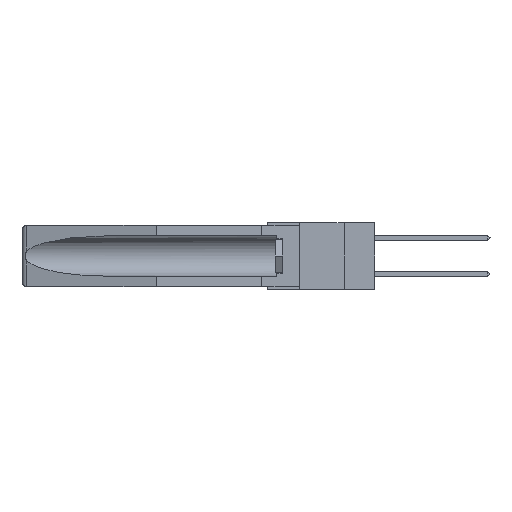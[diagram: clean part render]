
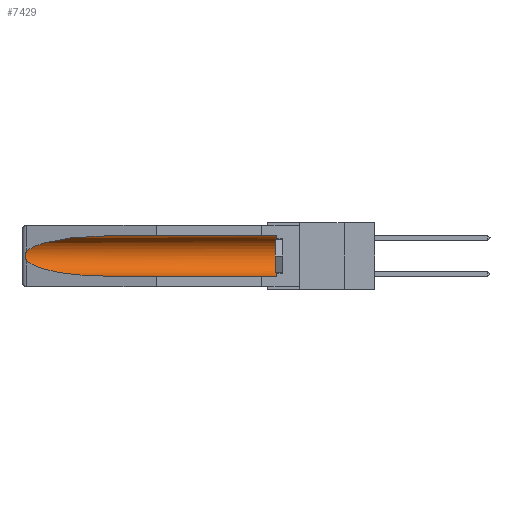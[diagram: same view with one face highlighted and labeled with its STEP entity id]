
A CAD part, left-side view. The second image highlights one B-rep face of the part: STEP entity #7429.
In plain terms, the highlighted cylindrical face has radius 2.857 mm (diameter 5.715 mm), a partial arc.
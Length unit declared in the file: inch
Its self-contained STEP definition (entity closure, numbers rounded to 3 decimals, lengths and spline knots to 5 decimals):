
#941 = DIRECTION ( 'NONE',  ( 0., 0., 1. ) ) ;
#954 = B_SPLINE_CURVE_WITH_KNOTS ( 'NONE', 3,
 ( #19045, #12262, #14741, #13070, #11184, #18297, #9565, #6142, #7768, #18066 ),
 .UNSPECIFIED., .F., .F.,
 ( 4, 2, 2, 2, 4 ),
 ( 0., 0.00029, 0.00058, 0.00087, 0.00117 ),
 .UNSPECIFIED. ) ;
#1592 = FACE_OUTER_BOUND ( 'NONE', #9227, .T. ) ;
#1776 = VECTOR ( 'NONE', #9390, 39.37008 ) ;
#2750 = CARTESIAN_POINT ( 'NONE',  ( 0.155, 0.126, -0.1715 ) ) ;
#2949 = CARTESIAN_POINT ( 'NONE',  ( 0.26537, 1.52718, -0.14972 ) ) ;
#3054 = DIRECTION ( 'NONE',  ( 0., 1., 0. ) ) ;
#3098 = CARTESIAN_POINT ( 'NONE',  ( 0.155, 1.07973, -0.059 ) ) ;
#4234 = DIRECTION ( 'NONE',  ( 0., -1., 0. ) ) ;
#4590 = CARTESIAN_POINT ( 'NONE',  ( 0.21114, 1.30732, -0.059 ) ) ;
#4625 = ORIENTED_EDGE ( 'NONE', *, *, #16347, .T. ) ;
#4761 = LINE ( 'NONE', #18281, #7692 ) ;
#4769 = CARTESIAN_POINT ( 'NONE',  ( 0.155, -0.30754, -0.1715 ) ) ;
#5114 = VERTEX_POINT ( 'NONE', #14726 ) ;
#5668 = VERTEX_POINT ( 'NONE', #7192 ) ;
#6033 =( BOUNDED_CURVE ( )  B_SPLINE_CURVE ( 3, ( #15786, #17613, #21273, #9541 ),
 .UNSPECIFIED., .F., .F. ) 
 B_SPLINE_CURVE_WITH_KNOTS ( ( 4, 4 ),
 ( 0.1948, 1.5708 ),
 .UNSPECIFIED. ) 
 CURVE ( )  GEOMETRIC_REPRESENTATION_ITEM ( )  RATIONAL_B_SPLINE_CURVE ( ( 1., 0.848, 0.848, 1. ) ) 
 REPRESENTATION_ITEM ( '' )  );
#6142 = CARTESIAN_POINT ( 'NONE',  ( 0.26655, 1.53094, -0.18657 ) ) ;
#6331 = LINE ( 'NONE', #19670, #1776 ) ;
#6953 = CYLINDRICAL_SURFACE ( 'NONE', #9958, 0.1125 ) ;
#7148 = CARTESIAN_POINT ( 'NONE',  ( 0.155, 0.126, -0.284 ) ) ;
#7192 = CARTESIAN_POINT ( 'NONE',  ( 0.155, 1.07973, -0.284 ) ) ;
#7429 = ADVANCED_FACE ( 'NONE', ( #1592 ), #6953, .F. ) ;
#7692 = VECTOR ( 'NONE', #7990, 39.37008 ) ;
#7768 = CARTESIAN_POINT ( 'NONE',  ( 0.26597, 1.5296, -0.19026 ) ) ;
#7795 = CIRCLE ( 'NONE', #7937, 0.1125 ) ;
#7937 = AXIS2_PLACEMENT_3D ( 'NONE', #2750, #4234, #941 ) ;
#7990 = DIRECTION ( 'NONE',  ( 0., 1., 0. ) ) ;
#8592 = CARTESIAN_POINT ( 'NONE',  ( 0.26537, 1.52718, -0.19328 ) ) ;
#8913 =( BOUNDED_CURVE ( )  B_SPLINE_CURVE ( 3, ( #9526, #4590, #18102, #2949 ),
 .UNSPECIFIED., .F., .F. ) 
 B_SPLINE_CURVE_WITH_KNOTS ( ( 4, 4 ),
 ( 4.71239, 6.08839 ),
 .UNSPECIFIED. ) 
 CURVE ( )  GEOMETRIC_REPRESENTATION_ITEM ( )  RATIONAL_B_SPLINE_CURVE ( ( 1., 0.848, 0.848, 1. ) ) 
 REPRESENTATION_ITEM ( '' )  );
#9115 = ORIENTED_EDGE ( 'NONE', *, *, #18691, .T. ) ;
#9195 = ORIENTED_EDGE ( 'NONE', *, *, #20794, .T. ) ;
#9227 = EDGE_LOOP ( 'NONE', ( #9115, #9195, #4625, #20875, #13393, #9527 ) ) ;
#9390 = DIRECTION ( 'NONE',  ( 0., 1., 0. ) ) ;
#9526 = CARTESIAN_POINT ( 'NONE',  ( 0.155, 1.07973, -0.059 ) ) ;
#9527 = ORIENTED_EDGE ( 'NONE', *, *, #21370, .T. ) ;
#9541 = CARTESIAN_POINT ( 'NONE',  ( 0.155, 1.07973, -0.284 ) ) ;
#9565 = CARTESIAN_POINT ( 'NONE',  ( 0.2673, 1.53269, -0.17917 ) ) ;
#9958 = AXIS2_PLACEMENT_3D ( 'NONE', #4769, #3054, #15026 ) ;
#9961 = EDGE_CURVE ( 'NONE', #12300, #5668, #6331, .T. ) ;
#10854 = VERTEX_POINT ( 'NONE', #3098 ) ;
#11184 = CARTESIAN_POINT ( 'NONE',  ( 0.2675, 1.53308, -0.16763 ) ) ;
#12178 = VERTEX_POINT ( 'NONE', #18484 ) ;
#12262 = CARTESIAN_POINT ( 'NONE',  ( 0.26597, 1.52961, -0.15275 ) ) ;
#12300 = VERTEX_POINT ( 'NONE', #7148 ) ;
#13070 = CARTESIAN_POINT ( 'NONE',  ( 0.2673, 1.5327, -0.16383 ) ) ;
#13393 = ORIENTED_EDGE ( 'NONE', *, *, #16386, .T. ) ;
#14726 = CARTESIAN_POINT ( 'NONE',  ( 0.26537, 1.52718, -0.14972 ) ) ;
#14741 = CARTESIAN_POINT ( 'NONE',  ( 0.26654, 1.53092, -0.15636 ) ) ;
#15026 = DIRECTION ( 'NONE',  ( 0., 0., 1. ) ) ;
#15786 = CARTESIAN_POINT ( 'NONE',  ( 0.26537, 1.52718, -0.19328 ) ) ;
#16347 = EDGE_CURVE ( 'NONE', #19656, #5668, #6033, .T. ) ;
#16386 = EDGE_CURVE ( 'NONE', #12300, #12178, #7795, .T. ) ;
#17613 = CARTESIAN_POINT ( 'NONE',  ( 0.25451, 1.48313, -0.24835 ) ) ;
#18066 = CARTESIAN_POINT ( 'NONE',  ( 0.26537, 1.52718, -0.19328 ) ) ;
#18102 = CARTESIAN_POINT ( 'NONE',  ( 0.25451, 1.48313, -0.09465 ) ) ;
#18281 = CARTESIAN_POINT ( 'NONE',  ( 0.155, -0.30754, -0.059 ) ) ;
#18297 = CARTESIAN_POINT ( 'NONE',  ( 0.2675, 1.53308, -0.17534 ) ) ;
#18484 = CARTESIAN_POINT ( 'NONE',  ( 0.155, 0.126, -0.059 ) ) ;
#18691 = EDGE_CURVE ( 'NONE', #10854, #5114, #8913, .T. ) ;
#19045 = CARTESIAN_POINT ( 'NONE',  ( 0.26537, 1.52718, -0.14972 ) ) ;
#19656 = VERTEX_POINT ( 'NONE', #8592 ) ;
#19670 = CARTESIAN_POINT ( 'NONE',  ( 0.155, -0.30754, -0.284 ) ) ;
#20794 = EDGE_CURVE ( 'NONE', #5114, #19656, #954, .T. ) ;
#20875 = ORIENTED_EDGE ( 'NONE', *, *, #9961, .F. ) ;
#21273 = CARTESIAN_POINT ( 'NONE',  ( 0.21114, 1.30732, -0.284 ) ) ;
#21370 = EDGE_CURVE ( 'NONE', #12178, #10854, #4761, .T. ) ;
